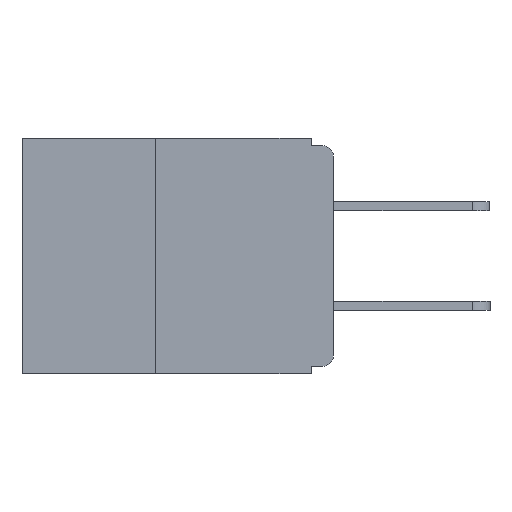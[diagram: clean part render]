
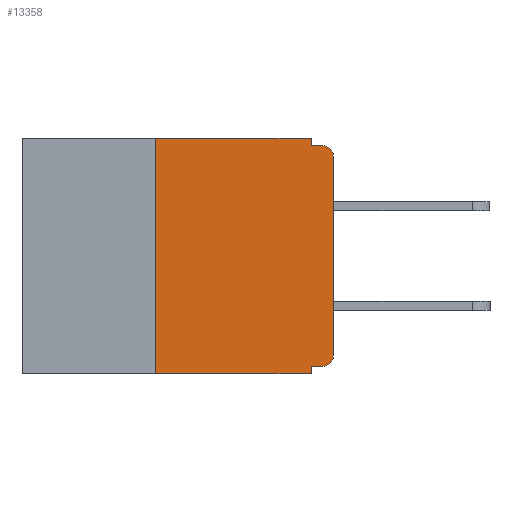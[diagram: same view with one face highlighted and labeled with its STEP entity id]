
A CAD part, left-side view. The second image highlights one B-rep face of the part: STEP entity #13358.
In plain terms, the highlighted planar face has unit normal (-1, 0, 0).
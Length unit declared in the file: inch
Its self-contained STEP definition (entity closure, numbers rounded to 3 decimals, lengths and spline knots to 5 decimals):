
#98 = AXIS2_PLACEMENT_3D ( 'NONE', #11984, #11966, #11926 ) ;
#268 = LINE ( 'NONE', #9928, #4360 ) ;
#346 = DIRECTION ( 'NONE',  ( 0., 0., 1. ) ) ;
#348 = VERTEX_POINT ( 'NONE', #14453 ) ;
#494 = DIRECTION ( 'NONE',  ( 0., 0., -1. ) ) ;
#1196 = CIRCLE ( 'NONE', #98, 0.015 ) ;
#1318 = VERTEX_POINT ( 'NONE', #8993 ) ;
#1622 = ORIENTED_EDGE ( 'NONE', *, *, #5878, .F. ) ;
#2253 = PLANE ( 'NONE',  #15423 ) ;
#2565 = EDGE_CURVE ( 'NONE', #14465, #10254, #1196, .T. ) ;
#2572 = VECTOR ( 'NONE', #10224, 39.37008 ) ;
#2765 = VECTOR ( 'NONE', #15290, 39.37008 ) ;
#3175 = ORIENTED_EDGE ( 'NONE', *, *, #4185, .T. ) ;
#3871 = EDGE_CURVE ( 'NONE', #1318, #9896, #12922, .T. ) ;
#3887 = LINE ( 'NONE', #8890, #2572 ) ;
#4185 = EDGE_CURVE ( 'NONE', #9896, #14465, #11402, .T. ) ;
#4360 = VECTOR ( 'NONE', #346, 39.37008 ) ;
#4388 = CARTESIAN_POINT ( 'NONE',  ( 0., 0.437, -0.33 ) ) ;
#4439 = EDGE_CURVE ( 'NONE', #348, #10926, #268, .T. ) ;
#4624 = DIRECTION ( 'NONE',  ( -1., 0., 0. ) ) ;
#4731 = VECTOR ( 'NONE', #494, 39.37008 ) ;
#5323 = VECTOR ( 'NONE', #5768, 39.37008 ) ;
#5768 = DIRECTION ( 'NONE',  ( 0., -1., 0. ) ) ;
#5801 = EDGE_CURVE ( 'NONE', #14756, #16608, #11135, .T. ) ;
#5802 = CARTESIAN_POINT ( 'NONE',  ( 0., 0.031, -0.33 ) ) ;
#5878 = EDGE_CURVE ( 'NONE', #1318, #12681, #3887, .T. ) ;
#6037 = CARTESIAN_POINT ( 'NONE',  ( 0., 0.031, 0. ) ) ;
#6109 = CARTESIAN_POINT ( 'NONE',  ( 0., 0.25, 0. ) ) ;
#6259 = VECTOR ( 'NONE', #7868, 39.37008 ) ;
#6646 = CARTESIAN_POINT ( 'NONE',  ( 0., 0., 0. ) ) ;
#7001 = EDGE_LOOP ( 'NONE', ( #3175, #10069, #15933, #13579, #13563, #9841, #8757, #13023, #1622, #13323 ) ) ;
#7183 = CARTESIAN_POINT ( 'NONE',  ( 0., 0.031, -0.33 ) ) ;
#7285 = LINE ( 'NONE', #7966, #10921 ) ;
#7764 = DIRECTION ( 'NONE',  ( 1., 0., 0. ) ) ;
#7868 = DIRECTION ( 'NONE',  ( 0., -1., 0. ) ) ;
#7966 = CARTESIAN_POINT ( 'NONE',  ( 0., 0.437, 0. ) ) ;
#8560 = LINE ( 'NONE', #4388, #5323 ) ;
#8757 = ORIENTED_EDGE ( 'NONE', *, *, #12456, .T. ) ;
#8890 = CARTESIAN_POINT ( 'NONE',  ( 0., 0., -0.32 ) ) ;
#8993 = CARTESIAN_POINT ( 'NONE',  ( 0., 0.015, -0.32 ) ) ;
#9841 = ORIENTED_EDGE ( 'NONE', *, *, #4439, .F. ) ;
#9896 = VERTEX_POINT ( 'NONE', #17481 ) ;
#9928 = CARTESIAN_POINT ( 'NONE',  ( 0., 0.25, -0.33 ) ) ;
#10069 = ORIENTED_EDGE ( 'NONE', *, *, #2565, .T. ) ;
#10224 = DIRECTION ( 'NONE',  ( 0., 1., 0. ) ) ;
#10254 = VERTEX_POINT ( 'NONE', #11494 ) ;
#10921 = VECTOR ( 'NONE', #16052, 39.37008 ) ;
#10926 = VERTEX_POINT ( 'NONE', #6109 ) ;
#11127 = EDGE_CURVE ( 'NONE', #10926, #14756, #7285, .T. ) ;
#11135 = LINE ( 'NONE', #14135, #4731 ) ;
#11402 = LINE ( 'NONE', #6646, #11849 ) ;
#11494 = CARTESIAN_POINT ( 'NONE',  ( 0., 0.015, -0.01 ) ) ;
#11849 = VECTOR ( 'NONE', #16126, 39.37008 ) ;
#11926 = DIRECTION ( 'NONE',  ( 0., 0., -1. ) ) ;
#11927 = CARTESIAN_POINT ( 'NONE',  ( 0., 0., -0.01 ) ) ;
#11966 = DIRECTION ( 'NONE',  ( -1., 0., 0. ) ) ;
#11984 = CARTESIAN_POINT ( 'NONE',  ( 0., 0.015, -0.025 ) ) ;
#12456 = EDGE_CURVE ( 'NONE', #348, #15844, #8560, .T. ) ;
#12681 = VERTEX_POINT ( 'NONE', #14430 ) ;
#12818 = CARTESIAN_POINT ( 'NONE',  ( 0., 0.015, -0.305 ) ) ;
#12922 = CIRCLE ( 'NONE', #13401, 0.015 ) ;
#13023 = ORIENTED_EDGE ( 'NONE', *, *, #16484, .F. ) ;
#13323 = ORIENTED_EDGE ( 'NONE', *, *, #3871, .T. ) ;
#13358 = ADVANCED_FACE ( 'NONE', ( #15450 ), #2253, .F. ) ;
#13401 = AXIS2_PLACEMENT_3D ( 'NONE', #12818, #4624, #14140 ) ;
#13563 = ORIENTED_EDGE ( 'NONE', *, *, #11127, .F. ) ;
#13579 = ORIENTED_EDGE ( 'NONE', *, *, #5801, .F. ) ;
#14135 = CARTESIAN_POINT ( 'NONE',  ( 0., 0.031, 0. ) ) ;
#14140 = DIRECTION ( 'NONE',  ( 0., 0., -1. ) ) ;
#14316 = CARTESIAN_POINT ( 'NONE',  ( 0., 0., -0.025 ) ) ;
#14430 = CARTESIAN_POINT ( 'NONE',  ( 0., 0.031, -0.32 ) ) ;
#14453 = CARTESIAN_POINT ( 'NONE',  ( 0., 0.25, -0.33 ) ) ;
#14465 = VERTEX_POINT ( 'NONE', #14316 ) ;
#14756 = VERTEX_POINT ( 'NONE', #6037 ) ;
#15290 = DIRECTION ( 'NONE',  ( 0., 0., -1. ) ) ;
#15423 = AXIS2_PLACEMENT_3D ( 'NONE', #15870, #7764, #17201 ) ;
#15450 = FACE_OUTER_BOUND ( 'NONE', #7001, .T. ) ;
#15496 = EDGE_CURVE ( 'NONE', #16608, #10254, #16202, .T. ) ;
#15844 = VERTEX_POINT ( 'NONE', #7183 ) ;
#15870 = CARTESIAN_POINT ( 'NONE',  ( 0., 0.437, 0. ) ) ;
#15933 = ORIENTED_EDGE ( 'NONE', *, *, #15496, .F. ) ;
#16052 = DIRECTION ( 'NONE',  ( 0., -1., 0. ) ) ;
#16126 = DIRECTION ( 'NONE',  ( 0., 0., 1. ) ) ;
#16202 = LINE ( 'NONE', #11927, #6259 ) ;
#16484 = EDGE_CURVE ( 'NONE', #12681, #15844, #17203, .T. ) ;
#16608 = VERTEX_POINT ( 'NONE', #16863 ) ;
#16863 = CARTESIAN_POINT ( 'NONE',  ( 0., 0.031, -0.01 ) ) ;
#17201 = DIRECTION ( 'NONE',  ( 0., 0., -1. ) ) ;
#17203 = LINE ( 'NONE', #5802, #2765 ) ;
#17481 = CARTESIAN_POINT ( 'NONE',  ( 0., 0., -0.305 ) ) ;
